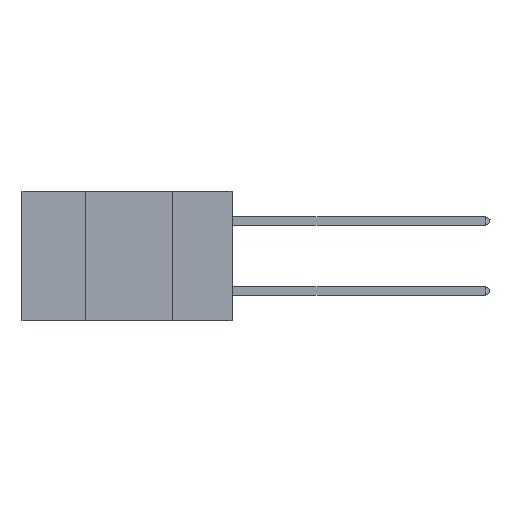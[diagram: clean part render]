
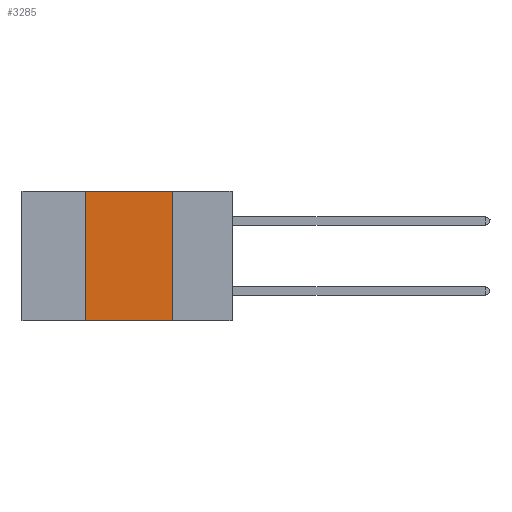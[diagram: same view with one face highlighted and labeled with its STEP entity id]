
A CAD part, left-side view. The second image highlights one B-rep face of the part: STEP entity #3285.
In plain terms, the highlighted planar face has unit normal (-1, 0, 0).
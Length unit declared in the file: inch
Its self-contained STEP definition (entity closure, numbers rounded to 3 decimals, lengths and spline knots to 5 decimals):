
#32 = PLANE ( 'NONE',  #1140 ) ;
#188 = DIRECTION ( 'NONE',  ( 1., 0., 0. ) ) ;
#323 = DIRECTION ( 'NONE',  ( 0., 0., 1. ) ) ;
#807 = FACE_OUTER_BOUND ( 'NONE', #8618, .T. ) ;
#1140 = AXIS2_PLACEMENT_3D ( 'NONE', #4200, #188, #13034 ) ;
#1180 = VECTOR ( 'NONE', #7066, 39.37008 ) ;
#1893 = CARTESIAN_POINT ( 'NONE',  ( 0., 0.6, 0. ) ) ;
#3285 = ADVANCED_FACE ( 'NONE', ( #807 ), #32, .F. ) ;
#3781 = CARTESIAN_POINT ( 'NONE',  ( 0., 0.42, -0.37 ) ) ;
#4199 = CARTESIAN_POINT ( 'NONE',  ( 0., 0.17, 0. ) ) ;
#4200 = CARTESIAN_POINT ( 'NONE',  ( 0., 0.6, 0. ) ) ;
#4598 = VECTOR ( 'NONE', #323, 39.37008 ) ;
#4989 = ORIENTED_EDGE ( 'NONE', *, *, #12805, .F. ) ;
#5147 = ORIENTED_EDGE ( 'NONE', *, *, #5766, .F. ) ;
#5150 = VECTOR ( 'NONE', #11347, 39.37008 ) ;
#5504 = ORIENTED_EDGE ( 'NONE', *, *, #8458, .F. ) ;
#5766 = EDGE_CURVE ( 'NONE', #9043, #11576, #9927, .T. ) ;
#6021 = CARTESIAN_POINT ( 'NONE',  ( 0., 0.6, -0.37 ) ) ;
#7008 = CARTESIAN_POINT ( 'NONE',  ( 0., 0.17, -0.37 ) ) ;
#7066 = DIRECTION ( 'NONE',  ( 0., -1., 0. ) ) ;
#7197 = VECTOR ( 'NONE', #11341, 39.37008 ) ;
#7645 = LINE ( 'NONE', #1893, #5150 ) ;
#7823 = ORIENTED_EDGE ( 'NONE', *, *, #10742, .T. ) ;
#8458 = EDGE_CURVE ( 'NONE', #8739, #9043, #7645, .T. ) ;
#8618 = EDGE_LOOP ( 'NONE', ( #5147, #5504, #4989, #7823 ) ) ;
#8739 = VERTEX_POINT ( 'NONE', #9800 ) ;
#8938 = CARTESIAN_POINT ( 'NONE',  ( 0., 0.42, 0. ) ) ;
#9043 = VERTEX_POINT ( 'NONE', #4199 ) ;
#9800 = CARTESIAN_POINT ( 'NONE',  ( 0., 0.42, 0. ) ) ;
#9927 = LINE ( 'NONE', #11374, #7197 ) ;
#10429 = LINE ( 'NONE', #8938, #4598 ) ;
#10742 = EDGE_CURVE ( 'NONE', #13389, #11576, #12395, .T. ) ;
#11341 = DIRECTION ( 'NONE',  ( 0., 0., -1. ) ) ;
#11347 = DIRECTION ( 'NONE',  ( 0., -1., 0. ) ) ;
#11374 = CARTESIAN_POINT ( 'NONE',  ( 0., 0.17, 0. ) ) ;
#11576 = VERTEX_POINT ( 'NONE', #7008 ) ;
#12395 = LINE ( 'NONE', #6021, #1180 ) ;
#12805 = EDGE_CURVE ( 'NONE', #13389, #8739, #10429, .T. ) ;
#13034 = DIRECTION ( 'NONE',  ( 0., 0., -1. ) ) ;
#13389 = VERTEX_POINT ( 'NONE', #3781 ) ;
